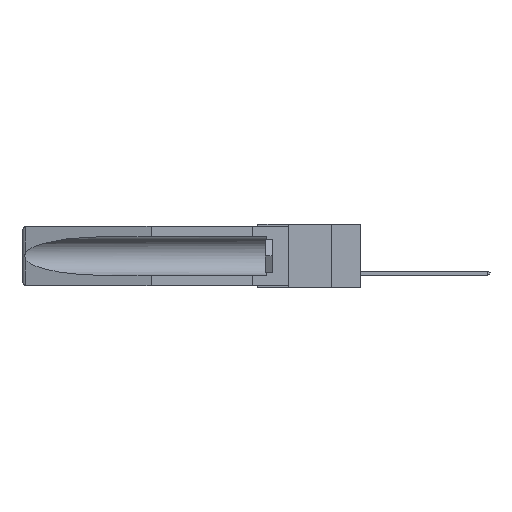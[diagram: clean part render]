
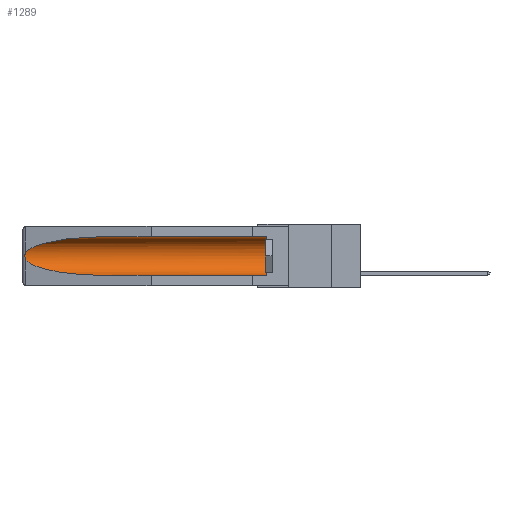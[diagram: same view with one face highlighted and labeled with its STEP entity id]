
A CAD part, left-side view. The second image highlights one B-rep face of the part: STEP entity #1289.
In plain terms, the highlighted cylindrical face has radius 2.857 mm (diameter 5.715 mm), a partial arc.
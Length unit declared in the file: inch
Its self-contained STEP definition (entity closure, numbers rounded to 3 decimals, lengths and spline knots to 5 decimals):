
#40 = CIRCLE ( 'NONE', #12430, 0.1125 ) ;
#297 = CARTESIAN_POINT ( 'NONE',  ( 0.26597, 1.52961, -0.15275 ) ) ;
#498 = EDGE_CURVE ( 'NONE', #4677, #11409, #1071, .T. ) ;
#915 = VERTEX_POINT ( 'NONE', #15736 ) ;
#1071 =( BOUNDED_CURVE ( )  B_SPLINE_CURVE ( 3, ( #5953, #17632, #2963, #16154 ),
 .UNSPECIFIED., .F., .F. ) 
 B_SPLINE_CURVE_WITH_KNOTS ( ( 4, 4 ),
 ( 4.71239, 6.08839 ),
 .UNSPECIFIED. ) 
 CURVE ( )  GEOMETRIC_REPRESENTATION_ITEM ( )  RATIONAL_B_SPLINE_CURVE ( ( 1., 0.848, 0.848, 1. ) ) 
 REPRESENTATION_ITEM ( '' )  );
#1289 = ADVANCED_FACE ( 'NONE', ( #14944 ), #11289, .F. ) ;
#1303 = CARTESIAN_POINT ( 'NONE',  ( 0.155, 1.07973, -0.284 ) ) ;
#1379 = ORIENTED_EDGE ( 'NONE', *, *, #9976, .T. ) ;
#1773 = CARTESIAN_POINT ( 'NONE',  ( 0.26537, 1.52718, -0.19328 ) ) ;
#2895 = DIRECTION ( 'NONE',  ( 0., 1., 0. ) ) ;
#2963 = CARTESIAN_POINT ( 'NONE',  ( 0.25451, 1.48313, -0.09465 ) ) ;
#2989 = CARTESIAN_POINT ( 'NONE',  ( 0.2673, 1.53269, -0.17917 ) ) ;
#3241 = CARTESIAN_POINT ( 'NONE',  ( 0.26537, 1.52718, -0.14972 ) ) ;
#3483 = DIRECTION ( 'NONE',  ( 0., 0., 1. ) ) ;
#3561 = CARTESIAN_POINT ( 'NONE',  ( 0.25451, 1.48313, -0.24835 ) ) ;
#3688 = ORIENTED_EDGE ( 'NONE', *, *, #16806, .T. ) ;
#4642 = CARTESIAN_POINT ( 'NONE',  ( 0.2675, 1.53308, -0.16763 ) ) ;
#4677 = VERTEX_POINT ( 'NONE', #5274 ) ;
#5030 = CARTESIAN_POINT ( 'NONE',  ( 0.155, 1.07973, -0.284 ) ) ;
#5274 = CARTESIAN_POINT ( 'NONE',  ( 0.155, 1.07973, -0.059 ) ) ;
#5299 = VERTEX_POINT ( 'NONE', #1303 ) ;
#5527 = ORIENTED_EDGE ( 'NONE', *, *, #498, .T. ) ;
#5806 = VERTEX_POINT ( 'NONE', #15719 ) ;
#5837 = VECTOR ( 'NONE', #11750, 39.37008 ) ;
#5851 = CARTESIAN_POINT ( 'NONE',  ( 0.26537, 1.52718, -0.14972 ) ) ;
#5953 = CARTESIAN_POINT ( 'NONE',  ( 0.155, 1.07973, -0.059 ) ) ;
#6363 = CARTESIAN_POINT ( 'NONE',  ( 0.21114, 1.30732, -0.284 ) ) ;
#7156 = CARTESIAN_POINT ( 'NONE',  ( 0.155, -0.30754, -0.059 ) ) ;
#7375 = CARTESIAN_POINT ( 'NONE',  ( 0.2673, 1.5327, -0.16383 ) ) ;
#7396 = EDGE_CURVE ( 'NONE', #12760, #5299, #12705, .T. ) ;
#7575 = CARTESIAN_POINT ( 'NONE',  ( 0.26597, 1.5296, -0.19026 ) ) ;
#8227 = LINE ( 'NONE', #7156, #15108 ) ;
#8766 = CARTESIAN_POINT ( 'NONE',  ( 0.155, -0.30754, -0.284 ) ) ;
#9239 =( BOUNDED_CURVE ( )  B_SPLINE_CURVE ( 3, ( #13805, #3561, #6363, #5030 ),
 .UNSPECIFIED., .F., .F. ) 
 B_SPLINE_CURVE_WITH_KNOTS ( ( 4, 4 ),
 ( 0.1948, 1.5708 ),
 .UNSPECIFIED. ) 
 CURVE ( )  GEOMETRIC_REPRESENTATION_ITEM ( )  RATIONAL_B_SPLINE_CURVE ( ( 1., 0.848, 0.848, 1. ) ) 
 REPRESENTATION_ITEM ( '' )  );
#9246 = CARTESIAN_POINT ( 'NONE',  ( 0.155, 0.126, -0.1715 ) ) ;
#9309 = DIRECTION ( 'NONE',  ( 0., 0., 1. ) ) ;
#9339 = CARTESIAN_POINT ( 'NONE',  ( 0.155, -0.30754, -0.1715 ) ) ;
#9391 = EDGE_LOOP ( 'NONE', ( #5527, #10010, #1379, #12912, #3688, #16333 ) ) ;
#9405 = DIRECTION ( 'NONE',  ( 0., 1., 0. ) ) ;
#9976 = EDGE_CURVE ( 'NONE', #5806, #5299, #9239, .T. ) ;
#10010 = ORIENTED_EDGE ( 'NONE', *, *, #10519, .T. ) ;
#10519 = EDGE_CURVE ( 'NONE', #11409, #5806, #12431, .T. ) ;
#10535 = CARTESIAN_POINT ( 'NONE',  ( 0.26655, 1.53094, -0.18657 ) ) ;
#11289 = CYLINDRICAL_SURFACE ( 'NONE', #11755, 0.1125 ) ;
#11409 = VERTEX_POINT ( 'NONE', #5851 ) ;
#11750 = DIRECTION ( 'NONE',  ( 0., 1., 0. ) ) ;
#11755 = AXIS2_PLACEMENT_3D ( 'NONE', #9339, #9405, #3483 ) ;
#11873 = CARTESIAN_POINT ( 'NONE',  ( 0.2675, 1.53308, -0.17534 ) ) ;
#12430 = AXIS2_PLACEMENT_3D ( 'NONE', #9246, #13752, #9309 ) ;
#12431 = B_SPLINE_CURVE_WITH_KNOTS ( 'NONE', 3,
 ( #3241, #297, #16116, #7375, #4642, #11873, #2989, #10535, #7575, #1773 ),
 .UNSPECIFIED., .F., .F.,
 ( 4, 2, 2, 2, 4 ),
 ( 0., 0.00029, 0.00058, 0.00087, 0.00117 ),
 .UNSPECIFIED. ) ;
#12705 = LINE ( 'NONE', #8766, #5837 ) ;
#12760 = VERTEX_POINT ( 'NONE', #13757 ) ;
#12912 = ORIENTED_EDGE ( 'NONE', *, *, #7396, .F. ) ;
#13752 = DIRECTION ( 'NONE',  ( 0., -1., 0. ) ) ;
#13757 = CARTESIAN_POINT ( 'NONE',  ( 0.155, 0.126, -0.284 ) ) ;
#13805 = CARTESIAN_POINT ( 'NONE',  ( 0.26537, 1.52718, -0.19328 ) ) ;
#14944 = FACE_OUTER_BOUND ( 'NONE', #9391, .T. ) ;
#15108 = VECTOR ( 'NONE', #2895, 39.37008 ) ;
#15719 = CARTESIAN_POINT ( 'NONE',  ( 0.26537, 1.52718, -0.19328 ) ) ;
#15736 = CARTESIAN_POINT ( 'NONE',  ( 0.155, 0.126, -0.059 ) ) ;
#16116 = CARTESIAN_POINT ( 'NONE',  ( 0.26654, 1.53092, -0.15636 ) ) ;
#16154 = CARTESIAN_POINT ( 'NONE',  ( 0.26537, 1.52718, -0.14972 ) ) ;
#16333 = ORIENTED_EDGE ( 'NONE', *, *, #18249, .T. ) ;
#16806 = EDGE_CURVE ( 'NONE', #12760, #915, #40, .T. ) ;
#17632 = CARTESIAN_POINT ( 'NONE',  ( 0.21114, 1.30732, -0.059 ) ) ;
#18249 = EDGE_CURVE ( 'NONE', #915, #4677, #8227, .T. ) ;
